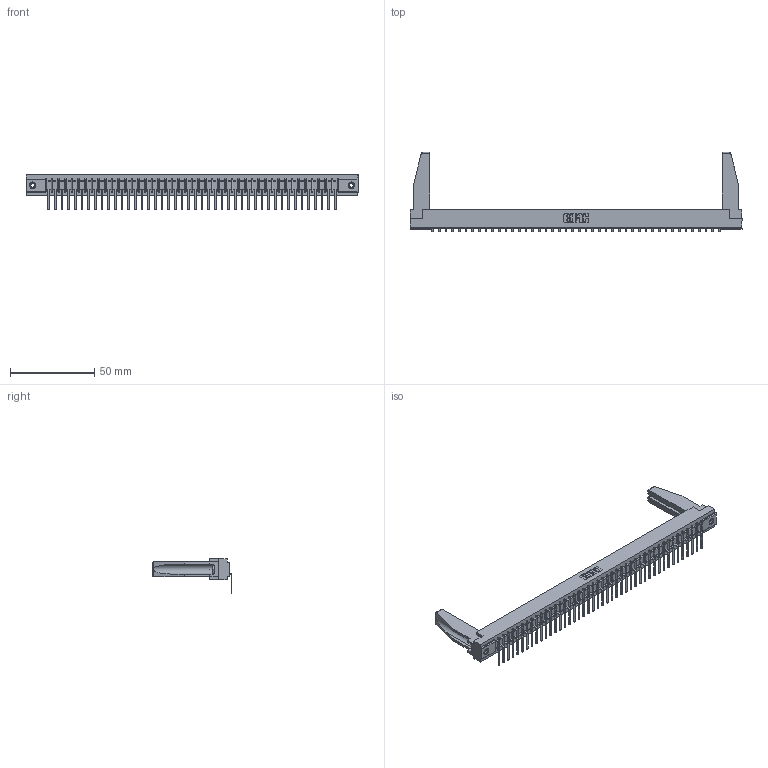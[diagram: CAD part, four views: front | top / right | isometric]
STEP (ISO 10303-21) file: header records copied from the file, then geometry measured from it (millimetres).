
FILE_DESCRIPTION (( 'STEP AP203' ), '1' );
FILE_NAME ('357-044-557-178.STEP', '2019-09-17T12:06:25', ( '' ), ( '' ), 'SwSTEP 2.0', 'SolidWorks 2016', '' );
FILE_SCHEMA (( 'CONFIG_CONTROL_DESIGN' ));
Length unit declared in the file: inch
Products named in the file (5): 307-220-078; 307-290-002_557; 307 Part_.156 Dia Mounting Holes; 345-250-001_345-250-001-102; 357-044-557-178
Assembly tree (49 placements, depth 2):
  357-044-557-178
    307 Part_.156 Dia Mounting Holes
    307-290-002_557  x44
    307-220-078  x2
    345-250-001_345-250-001-102  x2
Bounding box: 197.36 x 47.03 x 20.66 mm (x, y, z)
Volume: 25246.8 mm3; surface area: 31364 mm2
Topology: 49 solids, 49 shells, 3725 faces, 11389 edges, 7462 vertices
Faces by surface type: plane 2222, cylinder 1397, sphere 90, cone 12, torus 4
Entity records: 40767 total; most frequent: CARTESIAN_POINT 6878, ORIENTED_EDGE 6824, DIRECTION 6638, EDGE_CURVE 3412, LINE 2618, VECTOR 2618, VERTEX_POINT 2208, AXIS2_PLACEMENT_3D 2010
